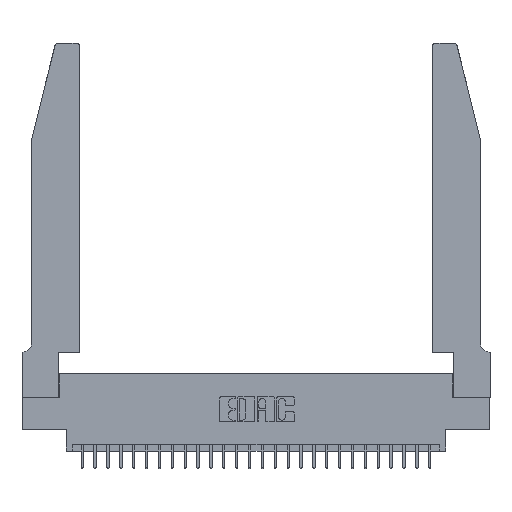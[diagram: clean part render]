
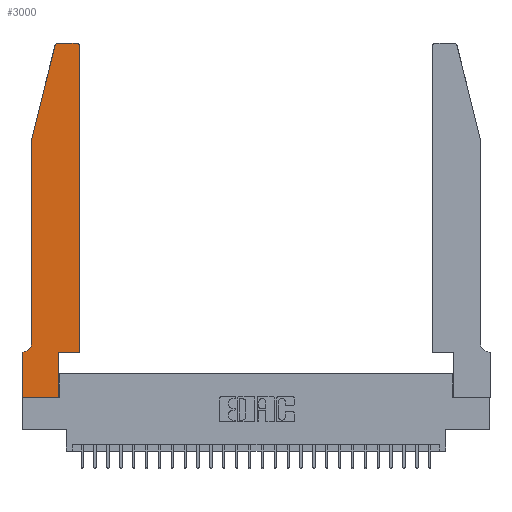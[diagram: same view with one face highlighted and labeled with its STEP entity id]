
A CAD part, top view. The second image highlights one B-rep face of the part: STEP entity #3000.
In plain terms, the highlighted planar face has unit normal (0, 0, 1).
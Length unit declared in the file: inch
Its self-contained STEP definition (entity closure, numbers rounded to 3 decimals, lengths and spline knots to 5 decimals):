
#78 = AXIS2_PLACEMENT_3D ( 'NONE', #27063, #17887, #15444 ) ;
#284 = LINE ( 'NONE', #2354, #16845 ) ;
#476 = ORIENTED_EDGE ( 'NONE', *, *, #23515, .T. ) ;
#608 = VECTOR ( 'NONE', #3114, 39.37008 ) ;
#1084 = VERTEX_POINT ( 'NONE', #17448 ) ;
#1240 = VECTOR ( 'NONE', #12670, 39.37008 ) ;
#1821 = VERTEX_POINT ( 'NONE', #17665 ) ;
#1960 = LINE ( 'NONE', #19727, #10358 ) ;
#2148 = DIRECTION ( 'NONE',  ( 0., 0., -1. ) ) ;
#2354 = CARTESIAN_POINT ( 'NONE',  ( 0., 0., 0.37 ) ) ;
#2396 = EDGE_CURVE ( 'NONE', #13345, #17885, #16297, .T. ) ;
#2430 = ORIENTED_EDGE ( 'NONE', *, *, #24398, .T. ) ;
#2634 = ORIENTED_EDGE ( 'NONE', *, *, #2396, .T. ) ;
#2895 = AXIS2_PLACEMENT_3D ( 'NONE', #11342, #11764, #20611 ) ;
#3000 = ADVANCED_FACE ( 'NONE', ( #8771 ), #24436, .T. ) ;
#3114 = DIRECTION ( 'NONE',  ( 1., 0., 0. ) ) ;
#3766 = CARTESIAN_POINT ( 'NONE',  ( 0.4205, 2.72, 0.37 ) ) ;
#3770 = CARTESIAN_POINT ( 'NONE',  ( 0.0055, 0.35, 0.37 ) ) ;
#3891 = DIRECTION ( 'NONE',  ( -1., 0., 0. ) ) ;
#4405 = VERTEX_POINT ( 'NONE', #19478 ) ;
#4657 = LINE ( 'NONE', #13706, #9369 ) ;
#4662 = DIRECTION ( 'NONE',  ( 1., 0., 0. ) ) ;
#4673 = CARTESIAN_POINT ( 'NONE',  ( 0.25487, 2.72718, 0.37 ) ) ;
#4849 = DIRECTION ( 'NONE',  ( 0., -1., 0. ) ) ;
#5082 = ORIENTED_EDGE ( 'NONE', *, *, #26213, .T. ) ;
#5697 = DIRECTION ( 'NONE',  ( -1., 0., 0. ) ) ;
#5957 = EDGE_CURVE ( 'NONE', #17764, #4405, #14218, .T. ) ;
#5986 = ORIENTED_EDGE ( 'NONE', *, *, #9013, .T. ) ;
#6256 = CARTESIAN_POINT ( 'NONE',  ( 0.4505, 0.35, 0.37 ) ) ;
#6284 = LINE ( 'NONE', #10623, #1240 ) ;
#6529 = DIRECTION ( 'NONE',  ( 0., 1., 0. ) ) ;
#7149 = DIRECTION ( 'NONE',  ( 0., 1., 0. ) ) ;
#7580 = EDGE_CURVE ( 'NONE', #21357, #16288, #4657, .T. ) ;
#7758 = ORIENTED_EDGE ( 'NONE', *, *, #22073, .T. ) ;
#8704 = ORIENTED_EDGE ( 'NONE', *, *, #16635, .T. ) ;
#8771 = FACE_OUTER_BOUND ( 'NONE', #21215, .T. ) ;
#9013 = EDGE_CURVE ( 'NONE', #18619, #1821, #284, .T. ) ;
#9369 = VECTOR ( 'NONE', #7149, 39.37008 ) ;
#9456 = ORIENTED_EDGE ( 'NONE', *, *, #13605, .T. ) ;
#9627 = CARTESIAN_POINT ( 'NONE',  ( 0.284, 2.75, 0.37 ) ) ;
#10188 = DIRECTION ( 'NONE',  ( 0., 0., 1. ) ) ;
#10358 = VECTOR ( 'NONE', #6529, 39.37008 ) ;
#10512 = CARTESIAN_POINT ( 'NONE',  ( 0.4505, 2.72, 0.37 ) ) ;
#10623 = CARTESIAN_POINT ( 'NONE',  ( 0.0755, 2., 0.37 ) ) ;
#10979 = VECTOR ( 'NONE', #5697, 39.37008 ) ;
#11342 = CARTESIAN_POINT ( 'NONE',  ( 0.284, 2.72, 0.37 ) ) ;
#11694 = VECTOR ( 'NONE', #4662, 39.37008 ) ;
#11764 = DIRECTION ( 'NONE',  ( 0., 0., 1. ) ) ;
#12621 = EDGE_CURVE ( 'NONE', #1821, #16394, #25105, .T. ) ;
#12670 = DIRECTION ( 'NONE',  ( 0., -1., 0. ) ) ;
#13345 = VERTEX_POINT ( 'NONE', #21511 ) ;
#13541 = CARTESIAN_POINT ( 'NONE',  ( 0.0055, 0.42, 0.37 ) ) ;
#13605 = EDGE_CURVE ( 'NONE', #21045, #18619, #18996, .T. ) ;
#13641 = AXIS2_PLACEMENT_3D ( 'NONE', #13541, #2148, #19903 ) ;
#13706 = CARTESIAN_POINT ( 'NONE',  ( 0.4505, 0.35, 0.37 ) ) ;
#14218 = LINE ( 'NONE', #16673, #26966 ) ;
#14358 = DIRECTION ( 'NONE',  ( -0.239, -0.971, 0. ) ) ;
#15444 = DIRECTION ( 'NONE',  ( 1., 0., 0. ) ) ;
#15510 = ORIENTED_EDGE ( 'NONE', *, *, #23313, .T. ) ;
#15517 = VERTEX_POINT ( 'NONE', #25010 ) ;
#16288 = VERTEX_POINT ( 'NONE', #10512 ) ;
#16297 = LINE ( 'NONE', #16725, #10979 ) ;
#16394 = VERTEX_POINT ( 'NONE', #20065 ) ;
#16635 = EDGE_CURVE ( 'NONE', #4405, #1084, #6284, .T. ) ;
#16673 = CARTESIAN_POINT ( 'NONE',  ( 0.0755, 2., 0.37 ) ) ;
#16725 = CARTESIAN_POINT ( 'NONE',  ( 0.2605, 2.75, 0.37 ) ) ;
#16845 = VECTOR ( 'NONE', #4849, 39.37008 ) ;
#16974 = VECTOR ( 'NONE', #3891, 39.37008 ) ;
#17448 = CARTESIAN_POINT ( 'NONE',  ( 0.0755, 0.42, 0.37 ) ) ;
#17665 = CARTESIAN_POINT ( 'NONE',  ( 0., 0., 0.37 ) ) ;
#17764 = VERTEX_POINT ( 'NONE', #4673 ) ;
#17885 = VERTEX_POINT ( 'NONE', #9627 ) ;
#17887 = DIRECTION ( 'NONE',  ( 0., 0., 1. ) ) ;
#17897 = LINE ( 'NONE', #24580, #11694 ) ;
#18399 = ORIENTED_EDGE ( 'NONE', *, *, #7580, .T. ) ;
#18619 = VERTEX_POINT ( 'NONE', #26717 ) ;
#18996 = LINE ( 'NONE', #23536, #16974 ) ;
#19478 = CARTESIAN_POINT ( 'NONE',  ( 0.0755, 2., 0.37 ) ) ;
#19727 = CARTESIAN_POINT ( 'NONE',  ( 0.2865, 0.35, 0.37 ) ) ;
#19903 = DIRECTION ( 'NONE',  ( -1., 0., 0. ) ) ;
#20065 = CARTESIAN_POINT ( 'NONE',  ( 0.2865, 0., 0.37 ) ) ;
#20611 = DIRECTION ( 'NONE',  ( 1., 0., 0. ) ) ;
#21045 = VERTEX_POINT ( 'NONE', #3770 ) ;
#21215 = EDGE_LOOP ( 'NONE', ( #2634, #15510, #23245, #8704, #2430, #9456, #5986, #26734, #476, #7758, #18399, #5082 ) ) ;
#21357 = VERTEX_POINT ( 'NONE', #6256 ) ;
#21483 = CIRCLE ( 'NONE', #2895, 0.03 ) ;
#21511 = CARTESIAN_POINT ( 'NONE',  ( 0.4205, 2.75, 0.37 ) ) ;
#22073 = EDGE_CURVE ( 'NONE', #15517, #21357, #17897, .T. ) ;
#22893 = CARTESIAN_POINT ( 'NONE',  ( 0., 0., 0.37 ) ) ;
#23245 = ORIENTED_EDGE ( 'NONE', *, *, #5957, .T. ) ;
#23313 = EDGE_CURVE ( 'NONE', #17885, #17764, #21483, .T. ) ;
#23515 = EDGE_CURVE ( 'NONE', #16394, #15517, #1960, .T. ) ;
#23536 = CARTESIAN_POINT ( 'NONE',  ( 0.0755, 0.35, 0.37 ) ) ;
#24398 = EDGE_CURVE ( 'NONE', #1084, #21045, #26180, .T. ) ;
#24436 = PLANE ( 'NONE',  #78 ) ;
#24580 = CARTESIAN_POINT ( 'NONE',  ( 0.4505, 0.35, 0.37 ) ) ;
#25010 = CARTESIAN_POINT ( 'NONE',  ( 0.2865, 0.35, 0.37 ) ) ;
#25105 = LINE ( 'NONE', #22893, #608 ) ;
#26180 = CIRCLE ( 'NONE', #13641, 0.07 ) ;
#26213 = EDGE_CURVE ( 'NONE', #16288, #13345, #26661, .T. ) ;
#26661 = CIRCLE ( 'NONE', #27572, 0.03 ) ;
#26717 = CARTESIAN_POINT ( 'NONE',  ( 0., 0.35, 0.37 ) ) ;
#26734 = ORIENTED_EDGE ( 'NONE', *, *, #12621, .T. ) ;
#26966 = VECTOR ( 'NONE', #14358, 39.37008 ) ;
#27063 = CARTESIAN_POINT ( 'NONE',  ( 0., 0.35, 0.37 ) ) ;
#27572 = AXIS2_PLACEMENT_3D ( 'NONE', #3766, #10188, #27653 ) ;
#27653 = DIRECTION ( 'NONE',  ( 1., 0., 0. ) ) ;
